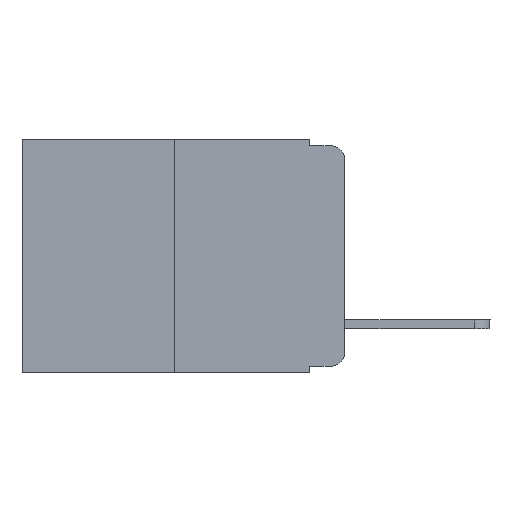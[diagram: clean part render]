
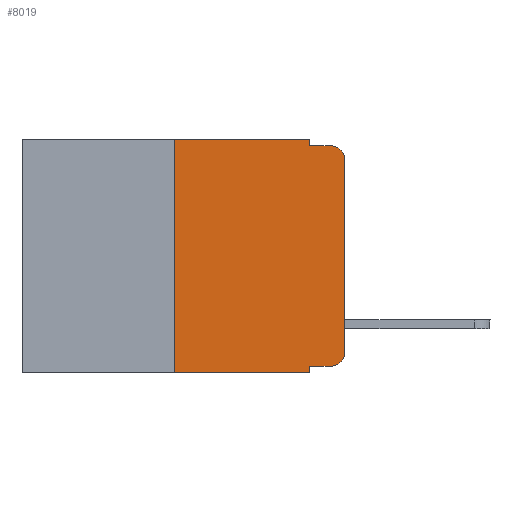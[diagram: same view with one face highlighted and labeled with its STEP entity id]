
A CAD part, left-side view. The second image highlights one B-rep face of the part: STEP entity #8019.
In plain terms, the highlighted planar face has unit normal (-1, 0, 0).
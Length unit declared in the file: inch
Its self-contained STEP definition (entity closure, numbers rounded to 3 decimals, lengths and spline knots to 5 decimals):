
#16 = DIRECTION ( 'NONE',  ( 0., 0., -1. ) ) ;
#502 = DIRECTION ( 'NONE',  ( 0., -1., 0. ) ) ;
#1946 = CARTESIAN_POINT ( 'NONE',  ( 0., 0.02, -0.313 ) ) ;
#2109 = CARTESIAN_POINT ( 'NONE',  ( 0., 0.051, -0.333 ) ) ;
#2205 = DIRECTION ( 'NONE',  ( -1., 0., 0. ) ) ;
#2320 = VERTEX_POINT ( 'NONE', #2109 ) ;
#2346 = CARTESIAN_POINT ( 'NONE',  ( 0., 0., 0. ) ) ;
#2686 = DIRECTION ( 'NONE',  ( -1., 0., 0. ) ) ;
#3080 = ORIENTED_EDGE ( 'NONE', *, *, #3694, .T. ) ;
#3213 = AXIS2_PLACEMENT_3D ( 'NONE', #1946, #2205, #15699 ) ;
#3341 = LINE ( 'NONE', #2346, #18008 ) ;
#3622 = ORIENTED_EDGE ( 'NONE', *, *, #22604, .F. ) ;
#3694 = EDGE_CURVE ( 'NONE', #24525, #18173, #21013, .T. ) ;
#3716 = CARTESIAN_POINT ( 'NONE',  ( 0., 0.051, -0.333 ) ) ;
#4309 = LINE ( 'NONE', #3716, #23511 ) ;
#4478 = CARTESIAN_POINT ( 'NONE',  ( 0., 0.02, -0.03 ) ) ;
#4528 = VERTEX_POINT ( 'NONE', #21023 ) ;
#4981 = EDGE_LOOP ( 'NONE', ( #6139, #19427, #12869, #19743, #23240, #3622, #3080, #11800, #9345, #22019 ) ) ;
#5231 = DIRECTION ( 'NONE',  ( 0., -1., 0. ) ) ;
#5456 = EDGE_CURVE ( 'NONE', #4528, #6640, #20639, .T. ) ;
#5755 = CARTESIAN_POINT ( 'NONE',  ( 0., 0.051, 0. ) ) ;
#6139 = ORIENTED_EDGE ( 'NONE', *, *, #20830, .T. ) ;
#6300 = AXIS2_PLACEMENT_3D ( 'NONE', #11520, #17068, #16 ) ;
#6332 = VERTEX_POINT ( 'NONE', #15200 ) ;
#6406 = EDGE_CURVE ( 'NONE', #2320, #18173, #18980, .T. ) ;
#6640 = VERTEX_POINT ( 'NONE', #6979 ) ;
#6979 = CARTESIAN_POINT ( 'NONE',  ( 0., 0.02, -0.01 ) ) ;
#7148 = CARTESIAN_POINT ( 'NONE',  ( 0., 0.25, -0.343 ) ) ;
#8019 = ADVANCED_FACE ( 'NONE', ( #19230 ), #21114, .F. ) ;
#8292 = VECTOR ( 'NONE', #20292, 39.37008 ) ;
#9080 = CARTESIAN_POINT ( 'NONE',  ( 0., 0.25, 0. ) ) ;
#9345 = ORIENTED_EDGE ( 'NONE', *, *, #19697, .T. ) ;
#10100 = CARTESIAN_POINT ( 'NONE',  ( 0., 0.051, 0. ) ) ;
#10884 = EDGE_CURVE ( 'NONE', #6332, #6640, #18479, .T. ) ;
#11324 = EDGE_CURVE ( 'NONE', #12671, #18234, #21497, .T. ) ;
#11333 = CARTESIAN_POINT ( 'NONE',  ( 0., 0., -0.313 ) ) ;
#11520 = CARTESIAN_POINT ( 'NONE',  ( 0., 0.473, 0. ) ) ;
#11800 = ORIENTED_EDGE ( 'NONE', *, *, #6406, .F. ) ;
#11805 = CARTESIAN_POINT ( 'NONE',  ( 0., 0.473, 0. ) ) ;
#12009 = DIRECTION ( 'NONE',  ( 0., 0., -1. ) ) ;
#12671 = VERTEX_POINT ( 'NONE', #24670 ) ;
#12869 = ORIENTED_EDGE ( 'NONE', *, *, #10884, .F. ) ;
#15200 = CARTESIAN_POINT ( 'NONE',  ( 0., 0.051, -0.01 ) ) ;
#15549 = AXIS2_PLACEMENT_3D ( 'NONE', #4478, #2686, #16087 ) ;
#15699 = DIRECTION ( 'NONE',  ( 0., 0., -1. ) ) ;
#15763 = CARTESIAN_POINT ( 'NONE',  ( 0., 0.051, 0. ) ) ;
#16087 = DIRECTION ( 'NONE',  ( 0., 0., -1. ) ) ;
#16324 = VECTOR ( 'NONE', #12009, 39.37008 ) ;
#17025 = LINE ( 'NONE', #5755, #17653 ) ;
#17068 = DIRECTION ( 'NONE',  ( 1., 0., 0. ) ) ;
#17653 = VECTOR ( 'NONE', #19145, 39.37008 ) ;
#17946 = CARTESIAN_POINT ( 'NONE',  ( 0., 0.051, -0.343 ) ) ;
#18008 = VECTOR ( 'NONE', #23519, 39.37008 ) ;
#18173 = VERTEX_POINT ( 'NONE', #17946 ) ;
#18234 = VERTEX_POINT ( 'NONE', #15763 ) ;
#18479 = LINE ( 'NONE', #24185, #8292 ) ;
#18936 = DIRECTION ( 'NONE',  ( 0., -1., 0. ) ) ;
#18980 = LINE ( 'NONE', #10100, #16324 ) ;
#19145 = DIRECTION ( 'NONE',  ( 0., 0., -1. ) ) ;
#19230 = FACE_OUTER_BOUND ( 'NONE', #4981, .T. ) ;
#19403 = VECTOR ( 'NONE', #22367, 39.37008 ) ;
#19427 = ORIENTED_EDGE ( 'NONE', *, *, #5456, .T. ) ;
#19515 = VECTOR ( 'NONE', #5231, 39.37008 ) ;
#19697 = EDGE_CURVE ( 'NONE', #2320, #20991, #4309, .T. ) ;
#19743 = ORIENTED_EDGE ( 'NONE', *, *, #22108, .F. ) ;
#20292 = DIRECTION ( 'NONE',  ( 0., -1., 0. ) ) ;
#20525 = EDGE_CURVE ( 'NONE', #20991, #24126, #23142, .T. ) ;
#20639 = CIRCLE ( 'NONE', #15549, 0.02 ) ;
#20830 = EDGE_CURVE ( 'NONE', #24126, #4528, #3341, .T. ) ;
#20991 = VERTEX_POINT ( 'NONE', #23223 ) ;
#21013 = LINE ( 'NONE', #22440, #19515 ) ;
#21023 = CARTESIAN_POINT ( 'NONE',  ( 0., 0., -0.03 ) ) ;
#21114 = PLANE ( 'NONE',  #6300 ) ;
#21497 = LINE ( 'NONE', #11805, #23306 ) ;
#22019 = ORIENTED_EDGE ( 'NONE', *, *, #20525, .T. ) ;
#22108 = EDGE_CURVE ( 'NONE', #18234, #6332, #17025, .T. ) ;
#22139 = LINE ( 'NONE', #9080, #19403 ) ;
#22367 = DIRECTION ( 'NONE',  ( 0., 0., 1. ) ) ;
#22440 = CARTESIAN_POINT ( 'NONE',  ( 0., 0.473, -0.343 ) ) ;
#22604 = EDGE_CURVE ( 'NONE', #24525, #12671, #22139, .T. ) ;
#23142 = CIRCLE ( 'NONE', #3213, 0.02 ) ;
#23223 = CARTESIAN_POINT ( 'NONE',  ( 0., 0.02, -0.333 ) ) ;
#23240 = ORIENTED_EDGE ( 'NONE', *, *, #11324, .F. ) ;
#23306 = VECTOR ( 'NONE', #502, 39.37008 ) ;
#23511 = VECTOR ( 'NONE', #18936, 39.37008 ) ;
#23519 = DIRECTION ( 'NONE',  ( 0., 0., 1. ) ) ;
#24126 = VERTEX_POINT ( 'NONE', #11333 ) ;
#24185 = CARTESIAN_POINT ( 'NONE',  ( 0., 0.051, -0.01 ) ) ;
#24525 = VERTEX_POINT ( 'NONE', #7148 ) ;
#24670 = CARTESIAN_POINT ( 'NONE',  ( 0., 0.25, 0. ) ) ;
